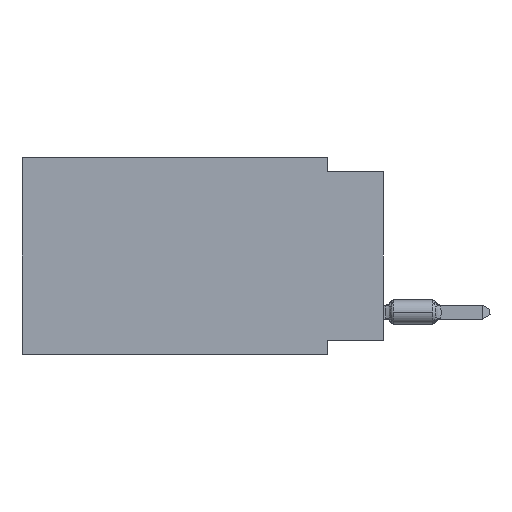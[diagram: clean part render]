
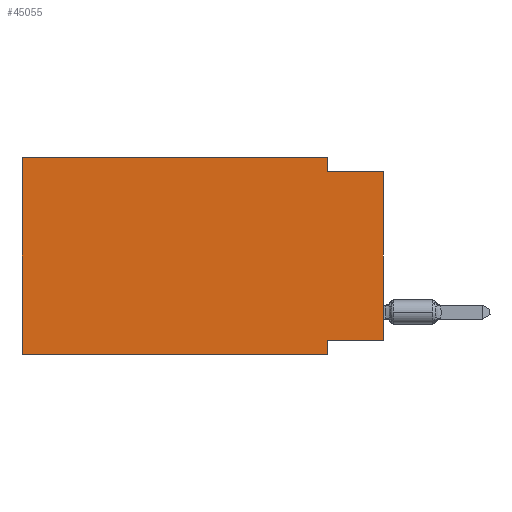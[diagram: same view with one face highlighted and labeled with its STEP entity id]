
A CAD part, left-side view. The second image highlights one B-rep face of the part: STEP entity #45055.
In plain terms, the highlighted planar face has unit normal (-1, 0, 0).
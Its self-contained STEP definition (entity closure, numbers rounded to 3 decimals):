
#911 = CARTESIAN_POINT ( 'NONE',  ( 0., 16.383, -8.89 ) ) ;
#2361 = PLANE ( 'NONE',  #46074 ) ;
#3351 = DIRECTION ( 'NONE',  ( 0., 0., 1. ) ) ;
#4268 = CARTESIAN_POINT ( 'NONE',  ( 0., 16.383, -8.89 ) ) ;
#5044 = LINE ( 'NONE', #15335, #15421 ) ;
#6001 = VECTOR ( 'NONE', #41170, 1000. ) ;
#8534 = VERTEX_POINT ( 'NONE', #65802 ) ;
#8607 = LINE ( 'NONE', #40501, #6001 ) ;
#11753 = VERTEX_POINT ( 'NONE', #53369 ) ;
#11843 = CARTESIAN_POINT ( 'NONE',  ( 0., 2.54, 0. ) ) ;
#11987 = CARTESIAN_POINT ( 'NONE',  ( 0., 2.54, -8.89 ) ) ;
#12575 = VECTOR ( 'NONE', #31671, 1000. ) ;
#13323 = DIRECTION ( 'NONE',  ( 1., 0., 0. ) ) ;
#13746 = VERTEX_POINT ( 'NONE', #64785 ) ;
#15335 = CARTESIAN_POINT ( 'NONE',  ( 0., 16.383, 0. ) ) ;
#15421 = VECTOR ( 'NONE', #25612, 1000. ) ;
#15511 = LINE ( 'NONE', #57377, #22069 ) ;
#17797 = FACE_OUTER_BOUND ( 'NONE', #37128, .T. ) ;
#17922 = VERTEX_POINT ( 'NONE', #911 ) ;
#18061 = CARTESIAN_POINT ( 'NONE',  ( 0., 2.54, 0. ) ) ;
#18450 = EDGE_CURVE ( 'NONE', #28059, #11753, #66124, .T. ) ;
#19804 = VECTOR ( 'NONE', #3351, 1000. ) ;
#20975 = EDGE_CURVE ( 'NONE', #17922, #40884, #67723, .T. ) ;
#21791 = VECTOR ( 'NONE', #59595, 1000. ) ;
#22069 = VECTOR ( 'NONE', #52548, 1000. ) ;
#22602 = VERTEX_POINT ( 'NONE', #11843 ) ;
#23497 = ORIENTED_EDGE ( 'NONE', *, *, #48258, .T. ) ;
#25142 = ORIENTED_EDGE ( 'NONE', *, *, #61269, .F. ) ;
#25612 = DIRECTION ( 'NONE',  ( 0., -1., 0. ) ) ;
#27878 = CARTESIAN_POINT ( 'NONE',  ( 0., 0., -0.635 ) ) ;
#28059 = VERTEX_POINT ( 'NONE', #60900 ) ;
#30391 = CARTESIAN_POINT ( 'NONE',  ( 0., 2.54, -8.89 ) ) ;
#30878 = VECTOR ( 'NONE', #44862, 1000. ) ;
#31119 = VECTOR ( 'NONE', #50995, 1000. ) ;
#31671 = DIRECTION ( 'NONE',  ( 0., -1., 0. ) ) ;
#34242 = DIRECTION ( 'NONE',  ( 0., 0., -1. ) ) ;
#34918 = CARTESIAN_POINT ( 'NONE',  ( 0., 16.383, 0. ) ) ;
#35656 = EDGE_CURVE ( 'NONE', #11753, #40884, #39347, .T. ) ;
#37128 = EDGE_LOOP ( 'NONE', ( #23497, #43397, #61810, #56018, #25142, #62148, #44946, #47125 ) ) ;
#39347 = LINE ( 'NONE', #30391, #31119 ) ;
#40501 = CARTESIAN_POINT ( 'NONE',  ( 0., 0., 0. ) ) ;
#40884 = VERTEX_POINT ( 'NONE', #11987 ) ;
#41170 = DIRECTION ( 'NONE',  ( 0., 0., 1. ) ) ;
#43397 = ORIENTED_EDGE ( 'NONE', *, *, #53365, .F. ) ;
#44862 = DIRECTION ( 'NONE',  ( 0., 1., 0. ) ) ;
#44946 = ORIENTED_EDGE ( 'NONE', *, *, #35656, .F. ) ;
#45055 = ADVANCED_FACE ( 'NONE', ( #17797 ), #2361, .F. ) ;
#46074 = AXIS2_PLACEMENT_3D ( 'NONE', #34918, #13323, #34242 ) ;
#47125 = ORIENTED_EDGE ( 'NONE', *, *, #18450, .F. ) ;
#48258 = EDGE_CURVE ( 'NONE', #28059, #60181, #8607, .T. ) ;
#49627 = LINE ( 'NONE', #18061, #21791 ) ;
#50331 = CARTESIAN_POINT ( 'NONE',  ( 0., 16.383, 0. ) ) ;
#50995 = DIRECTION ( 'NONE',  ( 0., 0., -1. ) ) ;
#52342 = EDGE_CURVE ( 'NONE', #13746, #22602, #5044, .T. ) ;
#52548 = DIRECTION ( 'NONE',  ( 0., -1., 0. ) ) ;
#53365 = EDGE_CURVE ( 'NONE', #8534, #60181, #15511, .T. ) ;
#53369 = CARTESIAN_POINT ( 'NONE',  ( 0., 2.54, -8.255 ) ) ;
#55827 = LINE ( 'NONE', #50331, #19804 ) ;
#56018 = ORIENTED_EDGE ( 'NONE', *, *, #52342, .F. ) ;
#57377 = CARTESIAN_POINT ( 'NONE',  ( 0., 0., -0.635 ) ) ;
#58994 = EDGE_CURVE ( 'NONE', #22602, #8534, #49627, .T. ) ;
#59595 = DIRECTION ( 'NONE',  ( 0., 0., -1. ) ) ;
#60181 = VERTEX_POINT ( 'NONE', #27878 ) ;
#60900 = CARTESIAN_POINT ( 'NONE',  ( 0., 0., -8.255 ) ) ;
#61269 = EDGE_CURVE ( 'NONE', #17922, #13746, #55827, .T. ) ;
#61810 = ORIENTED_EDGE ( 'NONE', *, *, #58994, .F. ) ;
#62148 = ORIENTED_EDGE ( 'NONE', *, *, #20975, .T. ) ;
#64785 = CARTESIAN_POINT ( 'NONE',  ( 0., 16.383, 0. ) ) ;
#65802 = CARTESIAN_POINT ( 'NONE',  ( 0., 2.54, -0.635 ) ) ;
#66124 = LINE ( 'NONE', #66454, #30878 ) ;
#66454 = CARTESIAN_POINT ( 'NONE',  ( 0., 0., -8.255 ) ) ;
#67723 = LINE ( 'NONE', #4268, #12575 ) ;
